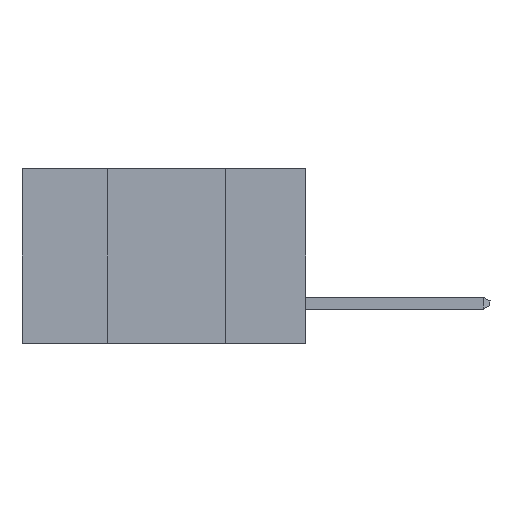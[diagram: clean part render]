
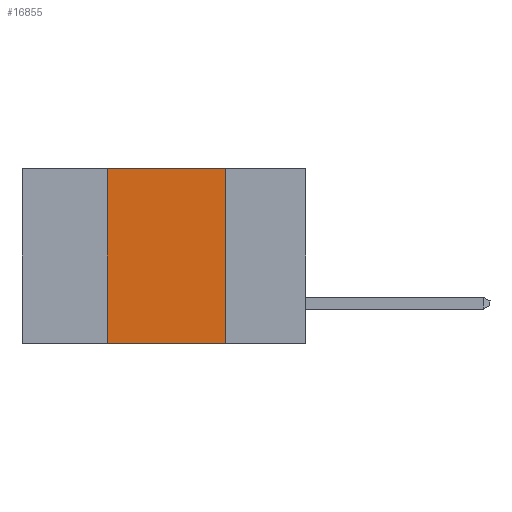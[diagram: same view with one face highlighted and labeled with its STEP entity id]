
A CAD part, left-side view. The second image highlights one B-rep face of the part: STEP entity #16855.
In plain terms, the highlighted planar face has unit normal (-1, 0, 0).
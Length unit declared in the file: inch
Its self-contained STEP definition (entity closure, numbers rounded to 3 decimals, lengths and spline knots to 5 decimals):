
#516 = CARTESIAN_POINT ( 'NONE',  ( 0., 0.42, -0.37 ) ) ;
#2019 = VERTEX_POINT ( 'NONE', #8370 ) ;
#2343 = ORIENTED_EDGE ( 'NONE', *, *, #22038, .T. ) ;
#3783 = LINE ( 'NONE', #516, #12876 ) ;
#3803 = CARTESIAN_POINT ( 'NONE',  ( 0., 0.17, -0.37 ) ) ;
#4899 = CARTESIAN_POINT ( 'NONE',  ( 0., 0.42, -0.37 ) ) ;
#5173 = DIRECTION ( 'NONE',  ( 0., 0., -1. ) ) ;
#5552 = CARTESIAN_POINT ( 'NONE',  ( 0., 0.6, 0. ) ) ;
#5662 = ORIENTED_EDGE ( 'NONE', *, *, #17849, .F. ) ;
#5826 = VERTEX_POINT ( 'NONE', #13400 ) ;
#6050 = EDGE_LOOP ( 'NONE', ( #13269, #18125, #5662, #2343 ) ) ;
#6369 = PLANE ( 'NONE',  #10707 ) ;
#6815 = DIRECTION ( 'NONE',  ( 0., 0., -1. ) ) ;
#7830 = LINE ( 'NONE', #16450, #17303 ) ;
#8370 = CARTESIAN_POINT ( 'NONE',  ( 0., 0.17, 0. ) ) ;
#9734 = DIRECTION ( 'NONE',  ( 0., -1., 0. ) ) ;
#10707 = AXIS2_PLACEMENT_3D ( 'NONE', #15111, #18484, #6815 ) ;
#12413 = EDGE_CURVE ( 'NONE', #5826, #2019, #13987, .T. ) ;
#12876 = VECTOR ( 'NONE', #14129, 39.37008 ) ;
#13223 = FACE_OUTER_BOUND ( 'NONE', #6050, .T. ) ;
#13269 = ORIENTED_EDGE ( 'NONE', *, *, #14595, .F. ) ;
#13338 = VECTOR ( 'NONE', #19153, 39.37008 ) ;
#13400 = CARTESIAN_POINT ( 'NONE',  ( 0., 0.42, 0. ) ) ;
#13987 = LINE ( 'NONE', #5552, #13338 ) ;
#14129 = DIRECTION ( 'NONE',  ( 0., 0., 1. ) ) ;
#14146 = LINE ( 'NONE', #3803, #21063 ) ;
#14595 = EDGE_CURVE ( 'NONE', #2019, #21935, #14146, .T. ) ;
#15111 = CARTESIAN_POINT ( 'NONE',  ( 0., 0.6, 0. ) ) ;
#16450 = CARTESIAN_POINT ( 'NONE',  ( 0., 0.6, -0.37 ) ) ;
#16855 = ADVANCED_FACE ( 'NONE', ( #13223 ), #6369, .F. ) ;
#17303 = VECTOR ( 'NONE', #9734, 39.37008 ) ;
#17849 = EDGE_CURVE ( 'NONE', #19484, #5826, #3783, .T. ) ;
#18125 = ORIENTED_EDGE ( 'NONE', *, *, #12413, .F. ) ;
#18484 = DIRECTION ( 'NONE',  ( 1., 0., 0. ) ) ;
#19153 = DIRECTION ( 'NONE',  ( 0., -1., 0. ) ) ;
#19484 = VERTEX_POINT ( 'NONE', #4899 ) ;
#19499 = CARTESIAN_POINT ( 'NONE',  ( 0., 0.17, -0.37 ) ) ;
#21063 = VECTOR ( 'NONE', #5173, 39.37008 ) ;
#21935 = VERTEX_POINT ( 'NONE', #19499 ) ;
#22038 = EDGE_CURVE ( 'NONE', #19484, #21935, #7830, .T. ) ;
